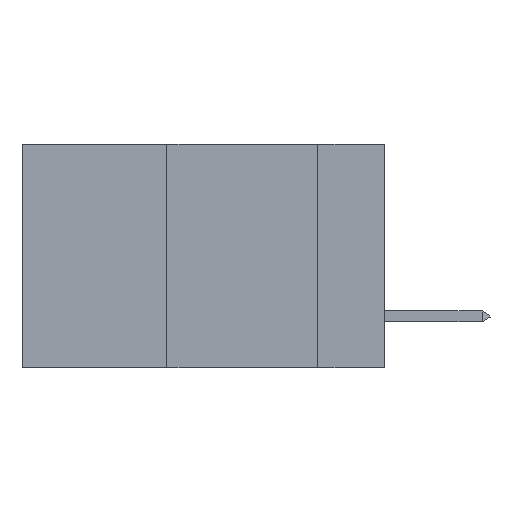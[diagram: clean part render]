
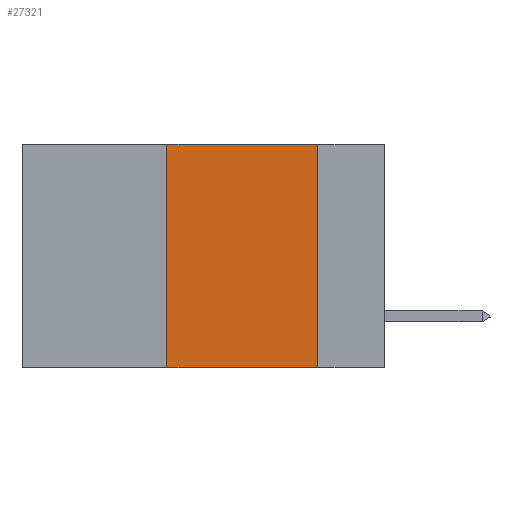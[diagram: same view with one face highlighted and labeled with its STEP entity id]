
A CAD part, left-side view. The second image highlights one B-rep face of the part: STEP entity #27321.
In plain terms, the highlighted planar face has unit normal (-1, 0, 0).
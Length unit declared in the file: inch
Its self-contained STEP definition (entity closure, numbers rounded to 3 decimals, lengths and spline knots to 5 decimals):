
#2992 = LINE ( 'NONE', #10669, #37940 ) ;
#5225 = EDGE_CURVE ( 'NONE', #30864, #18950, #35927, .T. ) ;
#6947 = EDGE_LOOP ( 'NONE', ( #38106, #8962, #11472, #9075 ) ) ;
#7332 = CARTESIAN_POINT ( 'NONE',  ( 0., 0.6, 0. ) ) ;
#8962 = ORIENTED_EDGE ( 'NONE', *, *, #19843, .F. ) ;
#9075 = ORIENTED_EDGE ( 'NONE', *, *, #32541, .T. ) ;
#9323 = LINE ( 'NONE', #23219, #49089 ) ;
#10669 = CARTESIAN_POINT ( 'NONE',  ( 0., 0.11, 0. ) ) ;
#11472 = ORIENTED_EDGE ( 'NONE', *, *, #5225, .F. ) ;
#15841 = VERTEX_POINT ( 'NONE', #31595 ) ;
#18236 = EDGE_CURVE ( 'NONE', #15841, #37194, #2992, .T. ) ;
#18947 = CARTESIAN_POINT ( 'NONE',  ( 0., 0.36, 0. ) ) ;
#18950 = VERTEX_POINT ( 'NONE', #18947 ) ;
#19643 = VECTOR ( 'NONE', #29666, 39.37008 ) ;
#19843 = EDGE_CURVE ( 'NONE', #18950, #15841, #27463, .T. ) ;
#20950 = CARTESIAN_POINT ( 'NONE',  ( 0., 0.36, -0.37 ) ) ;
#21935 = DIRECTION ( 'NONE',  ( 1., 0., 0. ) ) ;
#22032 = CARTESIAN_POINT ( 'NONE',  ( 0., 0.11, -0.37 ) ) ;
#23219 = CARTESIAN_POINT ( 'NONE',  ( 0., 0.6, -0.37 ) ) ;
#23445 = AXIS2_PLACEMENT_3D ( 'NONE', #7332, #21935, #48924 ) ;
#24423 = VECTOR ( 'NONE', #41626, 39.37008 ) ;
#24456 = FACE_OUTER_BOUND ( 'NONE', #6947, .T. ) ;
#26148 = PLANE ( 'NONE',  #23445 ) ;
#27321 = ADVANCED_FACE ( 'NONE', ( #24456 ), #26148, .F. ) ;
#27463 = LINE ( 'NONE', #40657, #19643 ) ;
#29666 = DIRECTION ( 'NONE',  ( 0., -1., 0. ) ) ;
#30864 = VERTEX_POINT ( 'NONE', #20950 ) ;
#31595 = CARTESIAN_POINT ( 'NONE',  ( 0., 0.11, 0. ) ) ;
#32541 = EDGE_CURVE ( 'NONE', #30864, #37194, #9323, .T. ) ;
#34704 = DIRECTION ( 'NONE',  ( 0., -1., 0. ) ) ;
#35927 = LINE ( 'NONE', #49841, #24423 ) ;
#37194 = VERTEX_POINT ( 'NONE', #22032 ) ;
#37642 = DIRECTION ( 'NONE',  ( 0., 0., -1. ) ) ;
#37940 = VECTOR ( 'NONE', #37642, 39.37008 ) ;
#38106 = ORIENTED_EDGE ( 'NONE', *, *, #18236, .F. ) ;
#40657 = CARTESIAN_POINT ( 'NONE',  ( 0., 0.6, 0. ) ) ;
#41626 = DIRECTION ( 'NONE',  ( 0., 0., 1. ) ) ;
#48924 = DIRECTION ( 'NONE',  ( 0., 0., -1. ) ) ;
#49089 = VECTOR ( 'NONE', #34704, 39.37008 ) ;
#49841 = CARTESIAN_POINT ( 'NONE',  ( 0., 0.36, 0. ) ) ;
